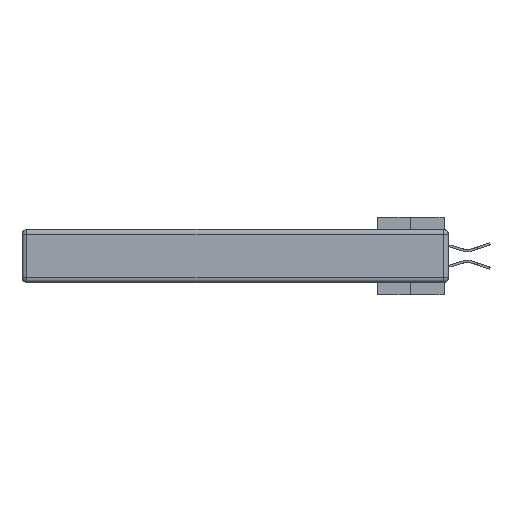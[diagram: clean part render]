
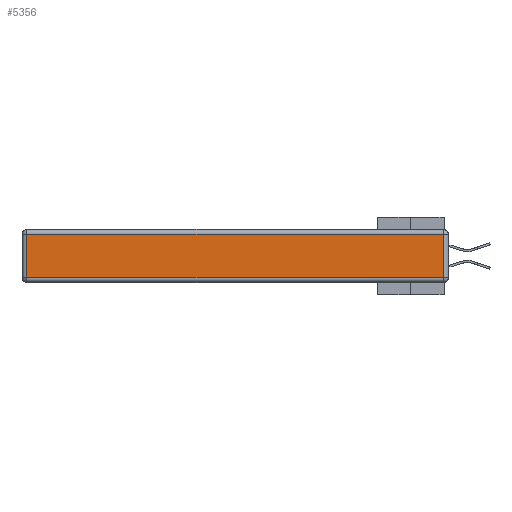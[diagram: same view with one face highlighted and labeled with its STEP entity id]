
A CAD part, left-side view. The second image highlights one B-rep face of the part: STEP entity #5356.
In plain terms, the highlighted planar face has unit normal (-1, 0, 0).
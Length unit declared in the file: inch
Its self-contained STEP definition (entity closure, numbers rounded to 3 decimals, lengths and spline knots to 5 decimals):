
#190 = ORIENTED_EDGE ( 'NONE', *, *, #18706, .T. ) ;
#478 = FACE_OUTER_BOUND ( 'NONE', #4601, .T. ) ;
#1227 = CARTESIAN_POINT ( 'NONE',  ( 0., 0.03, -0.313 ) ) ;
#4601 = EDGE_LOOP ( 'NONE', ( #18138, #190, #16431, #33496 ) ) ;
#5356 = ADVANCED_FACE ( 'NONE', ( #478 ), #29462, .T. ) ;
#5708 = VERTEX_POINT ( 'NONE', #29700 ) ;
#7142 = LINE ( 'NONE', #8107, #42335 ) ;
#7270 = LINE ( 'NONE', #24459, #45363 ) ;
#7307 = VECTOR ( 'NONE', #16849, 39.37008 ) ;
#7388 = CARTESIAN_POINT ( 'NONE',  ( 0., 0., -0.343 ) ) ;
#8107 = CARTESIAN_POINT ( 'NONE',  ( 0., 2.75, -0.03 ) ) ;
#12829 = DIRECTION ( 'NONE',  ( 0., -1., 0. ) ) ;
#14607 = EDGE_CURVE ( 'NONE', #30205, #5708, #7142, .T. ) ;
#14778 = DIRECTION ( 'NONE',  ( -1., 0., 0. ) ) ;
#16431 = ORIENTED_EDGE ( 'NONE', *, *, #14607, .T. ) ;
#16849 = DIRECTION ( 'NONE',  ( 0., 0., 1. ) ) ;
#18138 = ORIENTED_EDGE ( 'NONE', *, *, #29719, .T. ) ;
#18706 = EDGE_CURVE ( 'NONE', #44527, #30205, #36124, .T. ) ;
#21479 = CARTESIAN_POINT ( 'NONE',  ( 0., 2.72, -0.313 ) ) ;
#24459 = CARTESIAN_POINT ( 'NONE',  ( 0., 2.72, -0.343 ) ) ;
#25116 = DIRECTION ( 'NONE',  ( 0., 0., 1. ) ) ;
#25587 = AXIS2_PLACEMENT_3D ( 'NONE', #7388, #14778, #25116 ) ;
#27503 = CARTESIAN_POINT ( 'NONE',  ( 0., 0., -0.313 ) ) ;
#27974 = DIRECTION ( 'NONE',  ( 0., 0., -1. ) ) ;
#29462 = PLANE ( 'NONE',  #25587 ) ;
#29700 = CARTESIAN_POINT ( 'NONE',  ( 0., 2.72, -0.03 ) ) ;
#29719 = EDGE_CURVE ( 'NONE', #32857, #44527, #32361, .T. ) ;
#30205 = VERTEX_POINT ( 'NONE', #32017 ) ;
#32017 = CARTESIAN_POINT ( 'NONE',  ( 0., 0.03, -0.03 ) ) ;
#32361 = LINE ( 'NONE', #27503, #41019 ) ;
#32857 = VERTEX_POINT ( 'NONE', #21479 ) ;
#33496 = ORIENTED_EDGE ( 'NONE', *, *, #38129, .T. ) ;
#36124 = LINE ( 'NONE', #46081, #7307 ) ;
#37877 = DIRECTION ( 'NONE',  ( 0., 1., 0. ) ) ;
#38129 = EDGE_CURVE ( 'NONE', #5708, #32857, #7270, .T. ) ;
#41019 = VECTOR ( 'NONE', #12829, 39.37008 ) ;
#42335 = VECTOR ( 'NONE', #37877, 39.37008 ) ;
#44527 = VERTEX_POINT ( 'NONE', #1227 ) ;
#45363 = VECTOR ( 'NONE', #27974, 39.37008 ) ;
#46081 = CARTESIAN_POINT ( 'NONE',  ( 0., 0.03, -0.343 ) ) ;
